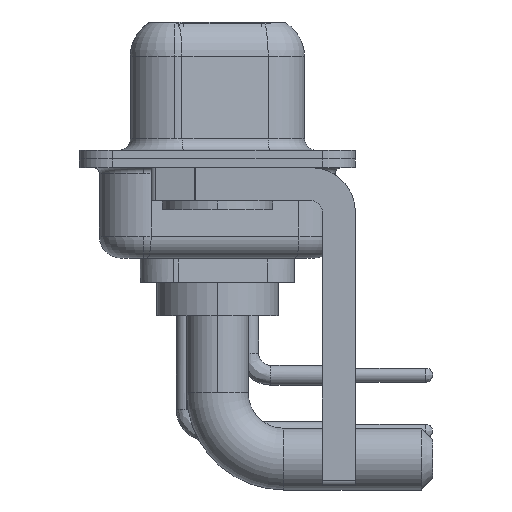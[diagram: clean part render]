
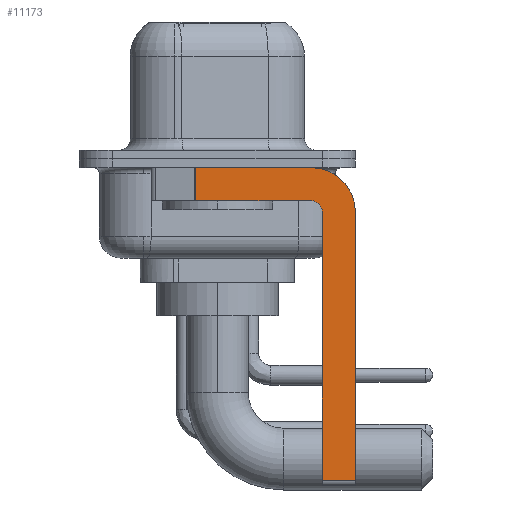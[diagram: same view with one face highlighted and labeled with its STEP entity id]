
A CAD part, left-side view. The second image highlights one B-rep face of the part: STEP entity #11173.
In plain terms, the highlighted planar face has unit normal (-1, 0, 0).
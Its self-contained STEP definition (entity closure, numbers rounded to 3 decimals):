
#71 = CARTESIAN_POINT ( 'NONE',  ( -2.9, 3., -0.4 ) ) ;
#115 = DIRECTION ( 'NONE',  ( 0., 0., -1. ) ) ;
#190 = CARTESIAN_POINT ( 'NONE',  ( -2.9, -4.25, -0.4 ) ) ;
#608 = ORIENTED_EDGE ( 'NONE', *, *, #11328, .F. ) ;
#694 = EDGE_CURVE ( 'NONE', #1381, #13692, #12506, .T. ) ;
#1381 = VERTEX_POINT ( 'NONE', #3888 ) ;
#1769 = ORIENTED_EDGE ( 'NONE', *, *, #17787, .F. ) ;
#1952 = ORIENTED_EDGE ( 'NONE', *, *, #14032, .F. ) ;
#2063 = EDGE_LOOP ( 'NONE', ( #15266, #4196, #9452, #608, #10208, #16877, #1769, #1952 ) ) ;
#2582 = FACE_OUTER_BOUND ( 'NONE', #2063, .T. ) ;
#3008 = CIRCLE ( 'NONE', #10588, 0.5 ) ;
#3204 = CARTESIAN_POINT ( 'NONE',  ( -2.9, -4.25, -2.4 ) ) ;
#3208 = LINE ( 'NONE', #14168, #7263 ) ;
#3320 = LINE ( 'NONE', #8893, #5106 ) ;
#3888 = CARTESIAN_POINT ( 'NONE',  ( -2.9, -4.25, -1.9 ) ) ;
#3986 = AXIS2_PLACEMENT_3D ( 'NONE', #11000, #8265, #13836 ) ;
#4196 = ORIENTED_EDGE ( 'NONE', *, *, #15687, .T. ) ;
#4318 = CARTESIAN_POINT ( 'NONE',  ( -2.9, 0.978, -1.9 ) ) ;
#4320 = DIRECTION ( 'NONE',  ( 1., 0., 0. ) ) ;
#4825 = VERTEX_POINT ( 'NONE', #190 ) ;
#4983 = CARTESIAN_POINT ( 'NONE',  ( -2.9, -4.75, -2.4 ) ) ;
#5095 = VECTOR ( 'NONE', #11191, 1000. ) ;
#5106 = VECTOR ( 'NONE', #14735, 1000. ) ;
#5160 = DIRECTION ( 'NONE',  ( 0., 0., -1. ) ) ;
#5346 = VERTEX_POINT ( 'NONE', #4983 ) ;
#5572 = CARTESIAN_POINT ( 'NONE',  ( -2.9, -4.25, -1.9 ) ) ;
#5775 = LINE ( 'NONE', #4318, #10729 ) ;
#6040 = DIRECTION ( 'NONE',  ( 0., 0., 1. ) ) ;
#6948 = VECTOR ( 'NONE', #5160, 1000. ) ;
#6983 = VERTEX_POINT ( 'NONE', #15045 ) ;
#7263 = VECTOR ( 'NONE', #10040, 1000. ) ;
#7677 = EDGE_CURVE ( 'NONE', #18025, #17816, #3320, .T. ) ;
#8156 = CARTESIAN_POINT ( 'NONE',  ( -2.9, -4.25, -2.4 ) ) ;
#8265 = DIRECTION ( 'NONE',  ( 1., 0., 0. ) ) ;
#8771 = DIRECTION ( 'NONE',  ( -1., 0., 0. ) ) ;
#8814 = LINE ( 'NONE', #71, #5095 ) ;
#8893 = CARTESIAN_POINT ( 'NONE',  ( -2.9, -4.25, -14.55 ) ) ;
#9310 = VERTEX_POINT ( 'NONE', #15053 ) ;
#9452 = ORIENTED_EDGE ( 'NONE', *, *, #694, .F. ) ;
#9864 = DIRECTION ( 'NONE',  ( 0., 0., -1. ) ) ;
#10040 = DIRECTION ( 'NONE',  ( 0., 0., 1. ) ) ;
#10208 = ORIENTED_EDGE ( 'NONE', *, *, #15162, .F. ) ;
#10588 = AXIS2_PLACEMENT_3D ( 'NONE', #3204, #8771, #6040 ) ;
#10668 = CIRCLE ( 'NONE', #3986, 2. ) ;
#10729 = VECTOR ( 'NONE', #9864, 1000. ) ;
#10919 = AXIS2_PLACEMENT_3D ( 'NONE', #8156, #4320, #115 ) ;
#11000 = CARTESIAN_POINT ( 'NONE',  ( -2.9, -4.25, -2.4 ) ) ;
#11173 = ADVANCED_FACE ( 'NONE', ( #2582 ), #15348, .F. ) ;
#11191 = DIRECTION ( 'NONE',  ( 0., -1., 0. ) ) ;
#11328 = EDGE_CURVE ( 'NONE', #5346, #1381, #3008, .T. ) ;
#12263 = EDGE_CURVE ( 'NONE', #9310, #4825, #8814, .T. ) ;
#12506 = LINE ( 'NONE', #5572, #13835 ) ;
#13692 = VERTEX_POINT ( 'NONE', #15735 ) ;
#13835 = VECTOR ( 'NONE', #16763, 1000. ) ;
#13836 = DIRECTION ( 'NONE',  ( 0., 0., -1. ) ) ;
#14032 = EDGE_CURVE ( 'NONE', #4825, #6983, #10668, .T. ) ;
#14073 = CARTESIAN_POINT ( 'NONE',  ( -2.9, -4.75, -14.55 ) ) ;
#14168 = CARTESIAN_POINT ( 'NONE',  ( -2.9, -4.75, -14.8 ) ) ;
#14735 = DIRECTION ( 'NONE',  ( 0., -1., 0. ) ) ;
#15045 = CARTESIAN_POINT ( 'NONE',  ( -2.9, -6.25, -2.4 ) ) ;
#15053 = CARTESIAN_POINT ( 'NONE',  ( -2.9, 0.978, -0.4 ) ) ;
#15162 = EDGE_CURVE ( 'NONE', #18025, #5346, #3208, .T. ) ;
#15266 = ORIENTED_EDGE ( 'NONE', *, *, #12263, .F. ) ;
#15348 = PLANE ( 'NONE',  #10919 ) ;
#15687 = EDGE_CURVE ( 'NONE', #9310, #13692, #5775, .T. ) ;
#15735 = CARTESIAN_POINT ( 'NONE',  ( -2.9, 0.978, -1.9 ) ) ;
#16076 = CARTESIAN_POINT ( 'NONE',  ( -2.9, -6.25, -14.55 ) ) ;
#16259 = CARTESIAN_POINT ( 'NONE',  ( -2.9, -6.25, -2.4 ) ) ;
#16763 = DIRECTION ( 'NONE',  ( 0., 1., 0. ) ) ;
#16877 = ORIENTED_EDGE ( 'NONE', *, *, #7677, .T. ) ;
#17633 = LINE ( 'NONE', #16259, #6948 ) ;
#17787 = EDGE_CURVE ( 'NONE', #6983, #17816, #17633, .T. ) ;
#17816 = VERTEX_POINT ( 'NONE', #16076 ) ;
#18025 = VERTEX_POINT ( 'NONE', #14073 ) ;
